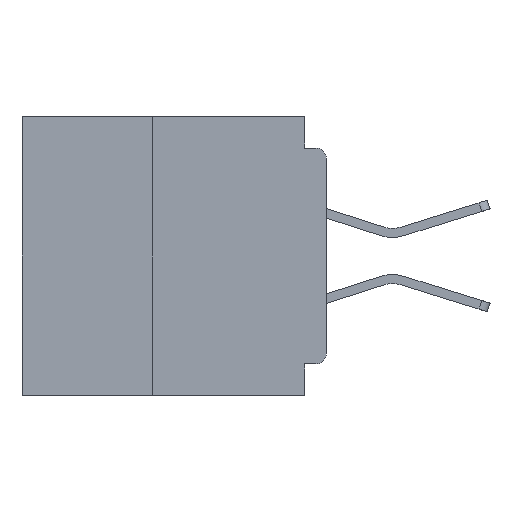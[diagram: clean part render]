
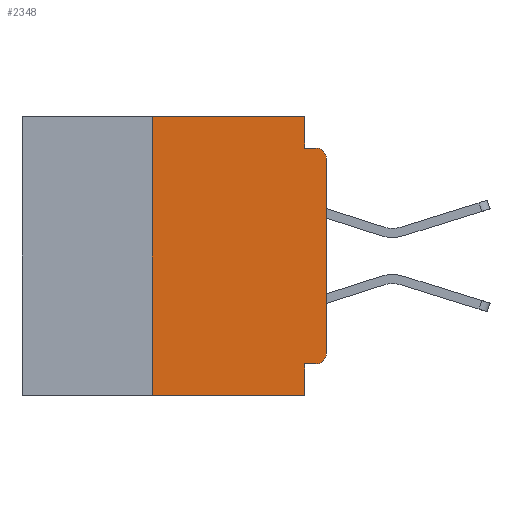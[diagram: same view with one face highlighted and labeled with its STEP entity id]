
A CAD part, left-side view. The second image highlights one B-rep face of the part: STEP entity #2348.
In plain terms, the highlighted planar face has unit normal (-1, 0, 0).
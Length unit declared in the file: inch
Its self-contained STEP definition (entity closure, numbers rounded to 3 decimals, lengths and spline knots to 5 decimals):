
#301 = EDGE_CURVE ( 'NONE', #21614, #35789, #28410, .T. ) ;
#543 = CARTESIAN_POINT ( 'NONE',  ( 0., 0., -0.355 ) ) ;
#1068 = LINE ( 'NONE', #26358, #15068 ) ;
#1507 = CARTESIAN_POINT ( 'NONE',  ( 0., 0.031, -0.4 ) ) ;
#2154 = CARTESIAN_POINT ( 'NONE',  ( 0., 0.031, -0.045 ) ) ;
#2348 = ADVANCED_FACE ( 'NONE', ( #35126 ), #31856, .F. ) ;
#3231 = DIRECTION ( 'NONE',  ( 0., 0., -1. ) ) ;
#4366 = DIRECTION ( 'NONE',  ( 0., 0., -1. ) ) ;
#4438 = AXIS2_PLACEMENT_3D ( 'NONE', #5006, #7597, #3231 ) ;
#4674 = EDGE_CURVE ( 'NONE', #30554, #13506, #27412, .T. ) ;
#4900 = EDGE_CURVE ( 'NONE', #13506, #24246, #35128, .T. ) ;
#5006 = CARTESIAN_POINT ( 'NONE',  ( 0., 0.437, 0. ) ) ;
#5638 = VERTEX_POINT ( 'NONE', #2154 ) ;
#5762 = VECTOR ( 'NONE', #14229, 39.37008 ) ;
#6003 = ORIENTED_EDGE ( 'NONE', *, *, #25224, .F. ) ;
#6276 = DIRECTION ( 'NONE',  ( -1., 0., 0. ) ) ;
#6290 = CARTESIAN_POINT ( 'NONE',  ( 0., 0.25, -0.4 ) ) ;
#6450 = DIRECTION ( 'NONE',  ( 0., 0., 1. ) ) ;
#6557 = VERTEX_POINT ( 'NONE', #11493 ) ;
#6686 = ORIENTED_EDGE ( 'NONE', *, *, #14693, .F. ) ;
#6969 = ORIENTED_EDGE ( 'NONE', *, *, #13531, .F. ) ;
#7023 = DIRECTION ( 'NONE',  ( 0., 0., -1. ) ) ;
#7256 = VECTOR ( 'NONE', #6450, 39.37008 ) ;
#7346 = ORIENTED_EDGE ( 'NONE', *, *, #301, .F. ) ;
#7597 = DIRECTION ( 'NONE',  ( 1., 0., 0. ) ) ;
#8958 = CARTESIAN_POINT ( 'NONE',  ( 0., 0.031, -0.4 ) ) ;
#9463 = EDGE_LOOP ( 'NONE', ( #34290, #31160, #6969, #6003, #19983, #7346, #16970, #23649, #6686, #12068 ) ) ;
#9476 = EDGE_CURVE ( 'NONE', #21614, #16780, #30989, .T. ) ;
#11493 = CARTESIAN_POINT ( 'NONE',  ( 0., 0.031, 0. ) ) ;
#11496 = CARTESIAN_POINT ( 'NONE',  ( 0., 0.25, -0.4 ) ) ;
#11797 = CARTESIAN_POINT ( 'NONE',  ( 0., 0.25, 0. ) ) ;
#11934 = CIRCLE ( 'NONE', #25095, 0.015 ) ;
#12068 = ORIENTED_EDGE ( 'NONE', *, *, #4674, .T. ) ;
#13281 = VECTOR ( 'NONE', #31676, 39.37008 ) ;
#13506 = VERTEX_POINT ( 'NONE', #28786 ) ;
#13531 = EDGE_CURVE ( 'NONE', #5638, #15679, #35255, .T. ) ;
#14044 = CARTESIAN_POINT ( 'NONE',  ( 0., 0., 0. ) ) ;
#14229 = DIRECTION ( 'NONE',  ( 0., 0., 1. ) ) ;
#14693 = EDGE_CURVE ( 'NONE', #30554, #35399, #33873, .T. ) ;
#15068 = VECTOR ( 'NONE', #7023, 39.37008 ) ;
#15679 = VERTEX_POINT ( 'NONE', #31222 ) ;
#16780 = VERTEX_POINT ( 'NONE', #8958 ) ;
#16970 = ORIENTED_EDGE ( 'NONE', *, *, #9476, .T. ) ;
#17550 = VECTOR ( 'NONE', #28336, 39.37008 ) ;
#17765 = DIRECTION ( 'NONE',  ( 0., 0., -1. ) ) ;
#17769 = DIRECTION ( 'NONE',  ( -1., 0., 0. ) ) ;
#17855 = CARTESIAN_POINT ( 'NONE',  ( 0., 0.015, -0.34 ) ) ;
#19904 = VECTOR ( 'NONE', #23013, 39.37008 ) ;
#19983 = ORIENTED_EDGE ( 'NONE', *, *, #35095, .F. ) ;
#20246 = CARTESIAN_POINT ( 'NONE',  ( 0., 0.437, 0. ) ) ;
#20603 = CARTESIAN_POINT ( 'NONE',  ( 0., 0., -0.06 ) ) ;
#21614 = VERTEX_POINT ( 'NONE', #11496 ) ;
#21848 = VECTOR ( 'NONE', #4366, 39.37008 ) ;
#21929 = CARTESIAN_POINT ( 'NONE',  ( 0., 0.031, -0.355 ) ) ;
#22788 = VECTOR ( 'NONE', #31443, 39.37008 ) ;
#22859 = CARTESIAN_POINT ( 'NONE',  ( 0., 0.015, -0.06 ) ) ;
#23013 = DIRECTION ( 'NONE',  ( 0., -1., 0. ) ) ;
#23579 = LINE ( 'NONE', #1507, #21848 ) ;
#23649 = ORIENTED_EDGE ( 'NONE', *, *, #26383, .F. ) ;
#24246 = VERTEX_POINT ( 'NONE', #20603 ) ;
#25095 = AXIS2_PLACEMENT_3D ( 'NONE', #22859, #6276, #25642 ) ;
#25224 = EDGE_CURVE ( 'NONE', #6557, #5638, #1068, .T. ) ;
#25605 = AXIS2_PLACEMENT_3D ( 'NONE', #17855, #17769, #17765 ) ;
#25642 = DIRECTION ( 'NONE',  ( 0., 0., -1. ) ) ;
#26358 = CARTESIAN_POINT ( 'NONE',  ( 0., 0.031, 0. ) ) ;
#26383 = EDGE_CURVE ( 'NONE', #35399, #16780, #23579, .T. ) ;
#27412 = CIRCLE ( 'NONE', #25605, 0.015 ) ;
#27502 = CARTESIAN_POINT ( 'NONE',  ( 0., 0.015, -0.355 ) ) ;
#28336 = DIRECTION ( 'NONE',  ( 0., 1., 0. ) ) ;
#28410 = LINE ( 'NONE', #6290, #7256 ) ;
#28670 = CARTESIAN_POINT ( 'NONE',  ( 0., 0.437, -0.4 ) ) ;
#28786 = CARTESIAN_POINT ( 'NONE',  ( 0., 0., -0.34 ) ) ;
#28904 = CARTESIAN_POINT ( 'NONE',  ( 0., 0., -0.045 ) ) ;
#30554 = VERTEX_POINT ( 'NONE', #27502 ) ;
#30989 = LINE ( 'NONE', #28670, #22788 ) ;
#31160 = ORIENTED_EDGE ( 'NONE', *, *, #31334, .T. ) ;
#31222 = CARTESIAN_POINT ( 'NONE',  ( 0., 0.015, -0.045 ) ) ;
#31334 = EDGE_CURVE ( 'NONE', #24246, #15679, #11934, .T. ) ;
#31443 = DIRECTION ( 'NONE',  ( 0., -1., 0. ) ) ;
#31676 = DIRECTION ( 'NONE',  ( 0., -1., 0. ) ) ;
#31856 = PLANE ( 'NONE',  #4438 ) ;
#33873 = LINE ( 'NONE', #543, #17550 ) ;
#34290 = ORIENTED_EDGE ( 'NONE', *, *, #4900, .T. ) ;
#34554 = LINE ( 'NONE', #20246, #19904 ) ;
#35095 = EDGE_CURVE ( 'NONE', #35789, #6557, #34554, .T. ) ;
#35126 = FACE_OUTER_BOUND ( 'NONE', #9463, .T. ) ;
#35128 = LINE ( 'NONE', #14044, #5762 ) ;
#35255 = LINE ( 'NONE', #28904, #13281 ) ;
#35399 = VERTEX_POINT ( 'NONE', #21929 ) ;
#35789 = VERTEX_POINT ( 'NONE', #11797 ) ;
